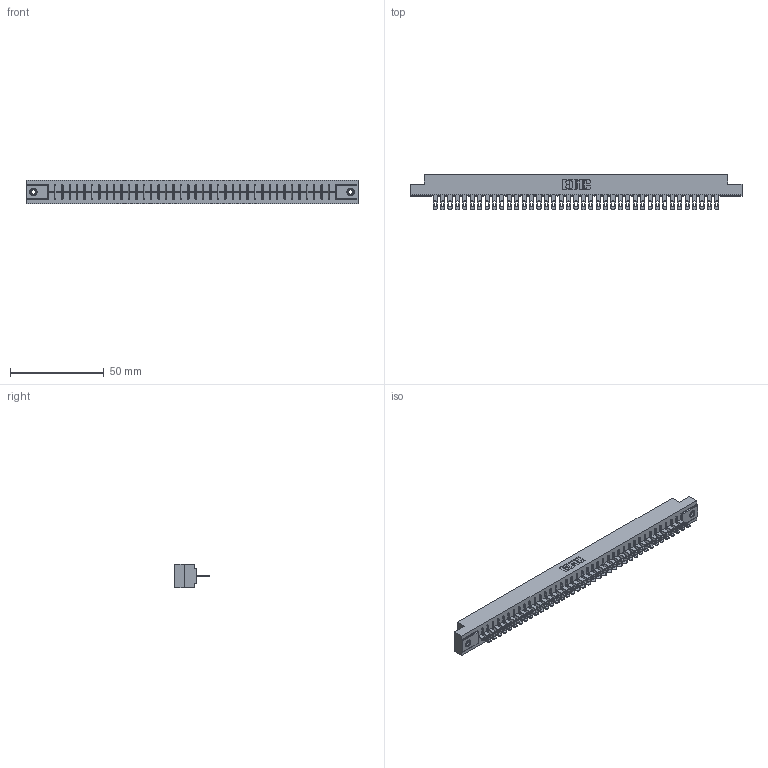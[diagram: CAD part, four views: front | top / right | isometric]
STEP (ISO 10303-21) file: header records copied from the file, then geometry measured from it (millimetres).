
FILE_DESCRIPTION (( 'STEP AP203' ), '1' );
FILE_NAME ('306-039-500-108.STEP', '2019-09-12T00:06:46', ( '' ), ( '' ), 'SwSTEP 2.0', 'SolidWorks 2016', '' );
FILE_SCHEMA (( 'CONFIG_CONTROL_DESIGN' ));
Length unit declared in the file: inch
Products named in the file (4): 306-290-001_100; 306-039-500-108; 306 Part_.156 Dia; 345-250-001_345-250-003-102
Assembly tree (42 placements, depth 2):
  306-039-500-108
    306 Part_.156 Dia
    306-290-001_100  x39
    345-250-001_345-250-003-102  x2
Bounding box: 177.55 x 18.87 x 12.7 mm (x, y, z)
Volume: 19725.7 mm3; surface area: 20927.2 mm2
Topology: 42 solids, 42 shells, 3140 faces, 8837 edges, 5674 vertices
Faces by surface type: plane 2050, cylinder 918, sphere 156, cone 12, torus 4
Entity records: 38107 total; most frequent: CARTESIAN_POINT 6379, ORIENTED_EDGE 6318, DIRECTION 6299, EDGE_CURVE 3159, LINE 2467, VECTOR 2467, VERTEX_POINT 1996, AXIS2_PLACEMENT_3D 1916
